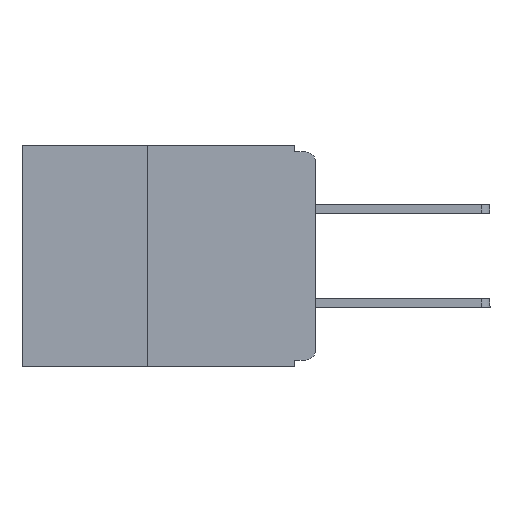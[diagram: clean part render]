
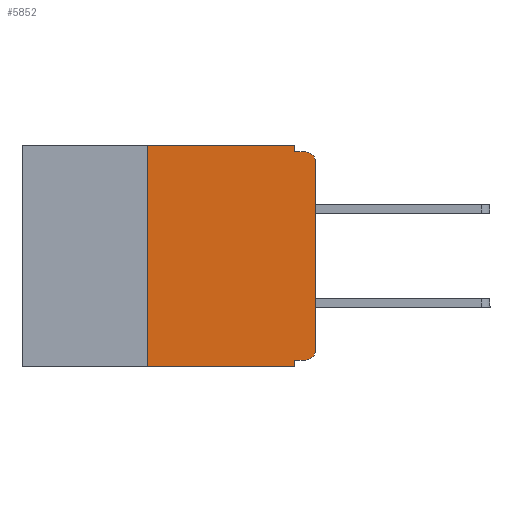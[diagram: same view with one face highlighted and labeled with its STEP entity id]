
A CAD part, left-side view. The second image highlights one B-rep face of the part: STEP entity #5852.
In plain terms, the highlighted planar face has unit normal (-1, 0, 0).
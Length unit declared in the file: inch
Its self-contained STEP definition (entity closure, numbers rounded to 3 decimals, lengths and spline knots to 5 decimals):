
#551 = VERTEX_POINT ( 'NONE', #16702 ) ;
#577 = CARTESIAN_POINT ( 'NONE',  ( 0., 0.015, -0.305 ) ) ;
#891 = EDGE_LOOP ( 'NONE', ( #11039, #12163, #2110, #16892, #6241, #8010, #19727, #15753, #1466, #11650 ) ) ;
#1043 = DIRECTION ( 'NONE',  ( 0., 0., 1. ) ) ;
#1125 = CARTESIAN_POINT ( 'NONE',  ( 0., 0.25, -0.33 ) ) ;
#1466 = ORIENTED_EDGE ( 'NONE', *, *, #18111, .F. ) ;
#1554 = EDGE_CURVE ( 'NONE', #5010, #551, #1580, .T. ) ;
#1580 = LINE ( 'NONE', #11664, #15442 ) ;
#1592 = CARTESIAN_POINT ( 'NONE',  ( 0., 0.25, -0.33 ) ) ;
#1834 = DIRECTION ( 'NONE',  ( 0., -1., 0. ) ) ;
#1905 = VERTEX_POINT ( 'NONE', #22510 ) ;
#2110 = ORIENTED_EDGE ( 'NONE', *, *, #16305, .F. ) ;
#2541 = DIRECTION ( 'NONE',  ( 0., 0., -1. ) ) ;
#2959 = CARTESIAN_POINT ( 'NONE',  ( 0., 0.031, -0.33 ) ) ;
#3203 = VECTOR ( 'NONE', #1043, 39.37008 ) ;
#3395 = CARTESIAN_POINT ( 'NONE',  ( 0., 0.031, 0. ) ) ;
#4446 = EDGE_CURVE ( 'NONE', #6223, #15882, #7676, .T. ) ;
#5010 = VERTEX_POINT ( 'NONE', #1592 ) ;
#5313 = CARTESIAN_POINT ( 'NONE',  ( 0., 0.031, -0.01 ) ) ;
#5852 = ADVANCED_FACE ( 'NONE', ( #11802 ), #21772, .F. ) ;
#6138 = LINE ( 'NONE', #19184, #10385 ) ;
#6223 = VERTEX_POINT ( 'NONE', #17886 ) ;
#6241 = ORIENTED_EDGE ( 'NONE', *, *, #14106, .F. ) ;
#6483 = LINE ( 'NONE', #16148, #15343 ) ;
#6704 = EDGE_CURVE ( 'NONE', #15882, #1905, #22359, .T. ) ;
#7029 = VECTOR ( 'NONE', #9946, 39.37008 ) ;
#7676 = LINE ( 'NONE', #14452, #20362 ) ;
#8010 = ORIENTED_EDGE ( 'NONE', *, *, #22650, .F. ) ;
#8186 = CARTESIAN_POINT ( 'NONE',  ( 0., 0.437, 0. ) ) ;
#9578 = CARTESIAN_POINT ( 'NONE',  ( 0., 0.031, -0.32 ) ) ;
#9946 = DIRECTION ( 'NONE',  ( 0., -1., 0. ) ) ;
#10348 = AXIS2_PLACEMENT_3D ( 'NONE', #12052, #12036, #12005 ) ;
#10385 = VECTOR ( 'NONE', #20850, 39.37008 ) ;
#10639 = DIRECTION ( 'NONE',  ( 0., -1., 0. ) ) ;
#11025 = AXIS2_PLACEMENT_3D ( 'NONE', #577, #13389, #2541 ) ;
#11039 = ORIENTED_EDGE ( 'NONE', *, *, #4446, .T. ) ;
#11628 = VERTEX_POINT ( 'NONE', #20073 ) ;
#11650 = ORIENTED_EDGE ( 'NONE', *, *, #20822, .T. ) ;
#11664 = CARTESIAN_POINT ( 'NONE',  ( 0., 0.437, -0.33 ) ) ;
#11802 = FACE_OUTER_BOUND ( 'NONE', #891, .T. ) ;
#11982 = VERTEX_POINT ( 'NONE', #5313 ) ;
#12005 = DIRECTION ( 'NONE',  ( 0., 0., -1. ) ) ;
#12036 = DIRECTION ( 'NONE',  ( -1., 0., 0. ) ) ;
#12052 = CARTESIAN_POINT ( 'NONE',  ( 0., 0.015, -0.025 ) ) ;
#12163 = ORIENTED_EDGE ( 'NONE', *, *, #6704, .T. ) ;
#13056 = VERTEX_POINT ( 'NONE', #17007 ) ;
#13389 = DIRECTION ( 'NONE',  ( -1., 0., 0. ) ) ;
#13782 = DIRECTION ( 'NONE',  ( 0., 0., -1. ) ) ;
#13854 = LINE ( 'NONE', #2959, #17873 ) ;
#14106 = EDGE_CURVE ( 'NONE', #11628, #22758, #20831, .T. ) ;
#14275 = DIRECTION ( 'NONE',  ( 0., 0., 1. ) ) ;
#14452 = CARTESIAN_POINT ( 'NONE',  ( 0., 0., 0. ) ) ;
#15142 = CARTESIAN_POINT ( 'NONE',  ( 0., 0., -0.025 ) ) ;
#15343 = VECTOR ( 'NONE', #1834, 39.37008 ) ;
#15442 = VECTOR ( 'NONE', #10639, 39.37008 ) ;
#15753 = ORIENTED_EDGE ( 'NONE', *, *, #19073, .F. ) ;
#15882 = VERTEX_POINT ( 'NONE', #15142 ) ;
#16148 = CARTESIAN_POINT ( 'NONE',  ( 0., 0., -0.01 ) ) ;
#16169 = CIRCLE ( 'NONE', #11025, 0.015 ) ;
#16289 = AXIS2_PLACEMENT_3D ( 'NONE', #21836, #21742, #21728 ) ;
#16305 = EDGE_CURVE ( 'NONE', #11982, #1905, #6483, .T. ) ;
#16702 = CARTESIAN_POINT ( 'NONE',  ( 0., 0.031, -0.33 ) ) ;
#16892 = ORIENTED_EDGE ( 'NONE', *, *, #22080, .F. ) ;
#17007 = CARTESIAN_POINT ( 'NONE',  ( 0., 0.015, -0.32 ) ) ;
#17040 = VERTEX_POINT ( 'NONE', #9578 ) ;
#17647 = LINE ( 'NONE', #19248, #21567 ) ;
#17873 = VECTOR ( 'NONE', #13782, 39.37008 ) ;
#17886 = CARTESIAN_POINT ( 'NONE',  ( 0., 0., -0.305 ) ) ;
#18111 = EDGE_CURVE ( 'NONE', #13056, #17040, #17647, .T. ) ;
#18476 = LINE ( 'NONE', #1125, #3203 ) ;
#19073 = EDGE_CURVE ( 'NONE', #17040, #551, #13854, .T. ) ;
#19184 = CARTESIAN_POINT ( 'NONE',  ( 0., 0.031, 0. ) ) ;
#19248 = CARTESIAN_POINT ( 'NONE',  ( 0., 0., -0.32 ) ) ;
#19727 = ORIENTED_EDGE ( 'NONE', *, *, #1554, .T. ) ;
#20073 = CARTESIAN_POINT ( 'NONE',  ( 0., 0.25, 0. ) ) ;
#20362 = VECTOR ( 'NONE', #14275, 39.37008 ) ;
#20822 = EDGE_CURVE ( 'NONE', #13056, #6223, #16169, .T. ) ;
#20831 = LINE ( 'NONE', #8186, #7029 ) ;
#20850 = DIRECTION ( 'NONE',  ( 0., 0., -1. ) ) ;
#20912 = DIRECTION ( 'NONE',  ( 0., 1., 0. ) ) ;
#21567 = VECTOR ( 'NONE', #20912, 39.37008 ) ;
#21728 = DIRECTION ( 'NONE',  ( 0., 0., -1. ) ) ;
#21742 = DIRECTION ( 'NONE',  ( 1., 0., 0. ) ) ;
#21772 = PLANE ( 'NONE',  #16289 ) ;
#21836 = CARTESIAN_POINT ( 'NONE',  ( 0., 0.437, 0. ) ) ;
#22080 = EDGE_CURVE ( 'NONE', #22758, #11982, #6138, .T. ) ;
#22359 = CIRCLE ( 'NONE', #10348, 0.015 ) ;
#22510 = CARTESIAN_POINT ( 'NONE',  ( 0., 0.015, -0.01 ) ) ;
#22650 = EDGE_CURVE ( 'NONE', #5010, #11628, #18476, .T. ) ;
#22758 = VERTEX_POINT ( 'NONE', #3395 ) ;
